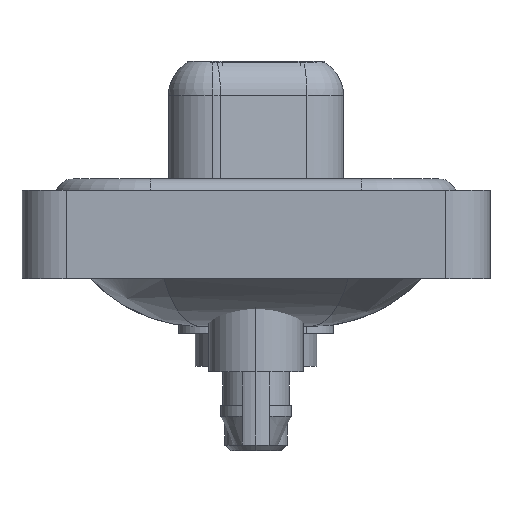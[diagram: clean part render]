
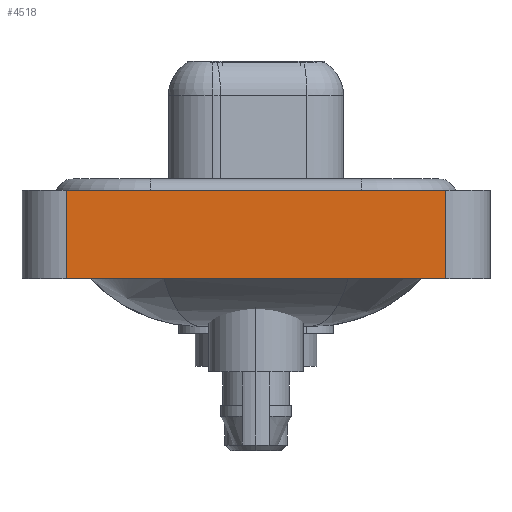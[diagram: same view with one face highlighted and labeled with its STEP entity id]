
A CAD part, left-side view. The second image highlights one B-rep face of the part: STEP entity #4518.
In plain terms, the highlighted planar face has unit normal (-1, 0, 0).
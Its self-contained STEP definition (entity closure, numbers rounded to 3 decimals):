
#128 = LINE ( 'NONE', #10253, #412 ) ;
#412 = VECTOR ( 'NONE', #13117, 1000. ) ;
#473 = DIRECTION ( 'NONE',  ( -1., 0., 0. ) ) ;
#1366 = PLANE ( 'NONE',  #11060 ) ;
#1431 = ORIENTED_EDGE ( 'NONE', *, *, #1549, .F. ) ;
#1549 = EDGE_CURVE ( 'NONE', #9650, #7141, #4018, .T. ) ;
#1611 = LINE ( 'NONE', #2974, #6998 ) ;
#1770 = VERTEX_POINT ( 'NONE', #16408 ) ;
#2021 = VECTOR ( 'NONE', #9193, 1000. ) ;
#2860 = CARTESIAN_POINT ( 'NONE',  ( -7.3, 8.55, 0.4 ) ) ;
#2974 = CARTESIAN_POINT ( 'NONE',  ( -7.3, -8.55, -3.6 ) ) ;
#3195 = LINE ( 'NONE', #14893, #12016 ) ;
#4018 = LINE ( 'NONE', #11667, #2021 ) ;
#4477 = CARTESIAN_POINT ( 'NONE',  ( -7.3, -8.55, -3.6 ) ) ;
#4518 = ADVANCED_FACE ( 'NONE', ( #12273 ), #1366, .T. ) ;
#6998 = VECTOR ( 'NONE', #7822, 1000. ) ;
#7026 = DIRECTION ( 'NONE',  ( 0., 0., 1. ) ) ;
#7141 = VERTEX_POINT ( 'NONE', #2860 ) ;
#7822 = DIRECTION ( 'NONE',  ( 0., -1., 0. ) ) ;
#8299 = EDGE_LOOP ( 'NONE', ( #9257, #14835, #1431, #9409 ) ) ;
#9193 = DIRECTION ( 'NONE',  ( 0., 0., 1. ) ) ;
#9257 = ORIENTED_EDGE ( 'NONE', *, *, #11745, .T. ) ;
#9409 = ORIENTED_EDGE ( 'NONE', *, *, #13283, .T. ) ;
#9523 = EDGE_CURVE ( 'NONE', #7141, #12831, #3195, .T. ) ;
#9545 = DIRECTION ( 'NONE',  ( 0., -1., 0. ) ) ;
#9650 = VERTEX_POINT ( 'NONE', #16529 ) ;
#10253 = CARTESIAN_POINT ( 'NONE',  ( -7.3, -8.55, -3.6 ) ) ;
#10303 = CARTESIAN_POINT ( 'NONE',  ( -7.3, -8.55, 0.4 ) ) ;
#11060 = AXIS2_PLACEMENT_3D ( 'NONE', #4477, #473, #7026 ) ;
#11667 = CARTESIAN_POINT ( 'NONE',  ( -7.3, 8.55, -3.6 ) ) ;
#11745 = EDGE_CURVE ( 'NONE', #1770, #12831, #128, .T. ) ;
#12016 = VECTOR ( 'NONE', #9545, 1000. ) ;
#12273 = FACE_OUTER_BOUND ( 'NONE', #8299, .T. ) ;
#12831 = VERTEX_POINT ( 'NONE', #10303 ) ;
#13117 = DIRECTION ( 'NONE',  ( 0., 0., 1. ) ) ;
#13283 = EDGE_CURVE ( 'NONE', #9650, #1770, #1611, .T. ) ;
#14835 = ORIENTED_EDGE ( 'NONE', *, *, #9523, .F. ) ;
#14893 = CARTESIAN_POINT ( 'NONE',  ( -7.3, -8.55, 0.4 ) ) ;
#16408 = CARTESIAN_POINT ( 'NONE',  ( -7.3, -8.55, -3.6 ) ) ;
#16529 = CARTESIAN_POINT ( 'NONE',  ( -7.3, 8.55, -3.6 ) ) ;
